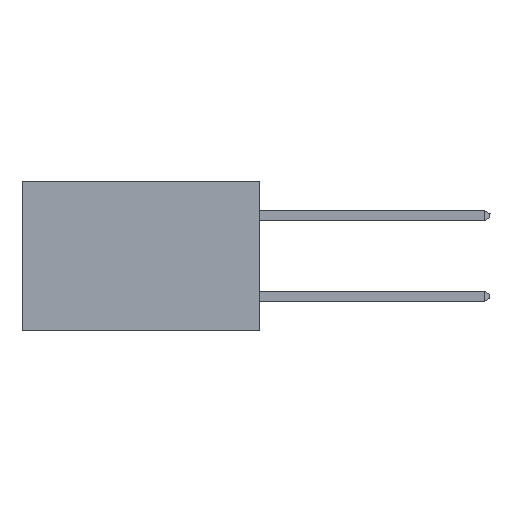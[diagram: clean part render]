
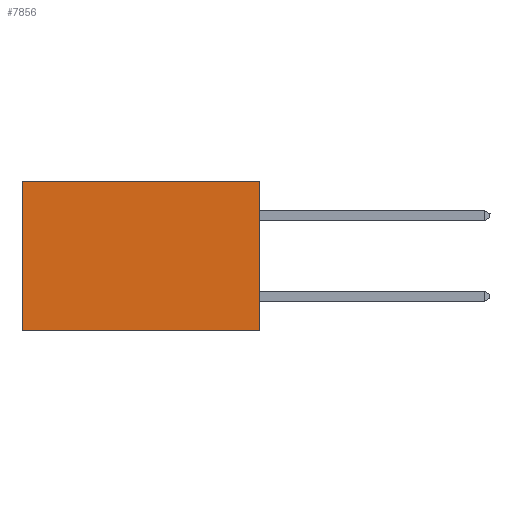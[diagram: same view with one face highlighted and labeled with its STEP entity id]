
A CAD part, left-side view. The second image highlights one B-rep face of the part: STEP entity #7856.
In plain terms, the highlighted planar face has unit normal (-1, 0, 0).
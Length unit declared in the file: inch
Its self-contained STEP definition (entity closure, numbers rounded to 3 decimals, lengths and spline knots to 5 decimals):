
#7 = DIRECTION ( 'NONE',  ( 0., 0., -1. ) ) ;
#23 = DIRECTION ( 'NONE',  ( 1., 0., 0. ) ) ;
#56 = EDGE_CURVE ( 'NONE', #6556, #1599, #856, .T. ) ;
#232 = CARTESIAN_POINT ( 'NONE',  ( 0.277, 0., -0.37 ) ) ;
#293 = PLANE ( 'NONE',  #1192 ) ;
#687 = DIRECTION ( 'NONE',  ( 0., 0., -1. ) ) ;
#711 = LINE ( 'NONE', #7963, #4978 ) ;
#856 = LINE ( 'NONE', #1538, #9437 ) ;
#989 = CARTESIAN_POINT ( 'NONE',  ( 0.277, 0.59, -0.37 ) ) ;
#1192 = AXIS2_PLACEMENT_3D ( 'NONE', #232, #23, #7 ) ;
#1538 = CARTESIAN_POINT ( 'NONE',  ( 0.277, 0.59, -0.37 ) ) ;
#1599 = VERTEX_POINT ( 'NONE', #989 ) ;
#1676 = EDGE_LOOP ( 'NONE', ( #5954, #6463, #7429, #2974 ) ) ;
#2760 = CARTESIAN_POINT ( 'NONE',  ( 0.277, 0.59, 0. ) ) ;
#2974 = ORIENTED_EDGE ( 'NONE', *, *, #8159, .T. ) ;
#3270 = CARTESIAN_POINT ( 'NONE',  ( 0.277, 0., -0.37 ) ) ;
#3379 = LINE ( 'NONE', #5801, #9681 ) ;
#3879 = VERTEX_POINT ( 'NONE', #10539 ) ;
#4040 = FACE_OUTER_BOUND ( 'NONE', #1676, .T. ) ;
#4437 = LINE ( 'NONE', #6670, #10642 ) ;
#4978 = VECTOR ( 'NONE', #8092, 39.37008 ) ;
#5801 = CARTESIAN_POINT ( 'NONE',  ( 0.277, 0., 0. ) ) ;
#5954 = ORIENTED_EDGE ( 'NONE', *, *, #56, .T. ) ;
#6463 = ORIENTED_EDGE ( 'NONE', *, *, #7537, .F. ) ;
#6556 = VERTEX_POINT ( 'NONE', #2760 ) ;
#6631 = DIRECTION ( 'NONE',  ( 0., 1., 0. ) ) ;
#6670 = CARTESIAN_POINT ( 'NONE',  ( 0.277, 0., -0.37 ) ) ;
#7429 = ORIENTED_EDGE ( 'NONE', *, *, #7452, .F. ) ;
#7441 = DIRECTION ( 'NONE',  ( 0., 1., 0. ) ) ;
#7452 = EDGE_CURVE ( 'NONE', #3879, #7747, #711, .T. ) ;
#7537 = EDGE_CURVE ( 'NONE', #7747, #1599, #4437, .T. ) ;
#7747 = VERTEX_POINT ( 'NONE', #3270 ) ;
#7856 = ADVANCED_FACE ( 'NONE', ( #4040 ), #293, .F. ) ;
#7963 = CARTESIAN_POINT ( 'NONE',  ( 0.277, 0., -0.37 ) ) ;
#8092 = DIRECTION ( 'NONE',  ( 0., 0., -1. ) ) ;
#8159 = EDGE_CURVE ( 'NONE', #3879, #6556, #3379, .T. ) ;
#9437 = VECTOR ( 'NONE', #687, 39.37008 ) ;
#9681 = VECTOR ( 'NONE', #7441, 39.37008 ) ;
#10539 = CARTESIAN_POINT ( 'NONE',  ( 0.277, 0., 0. ) ) ;
#10642 = VECTOR ( 'NONE', #6631, 39.37008 ) ;
